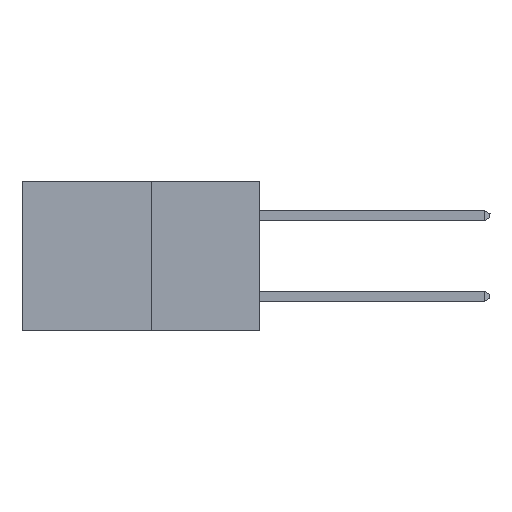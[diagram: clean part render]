
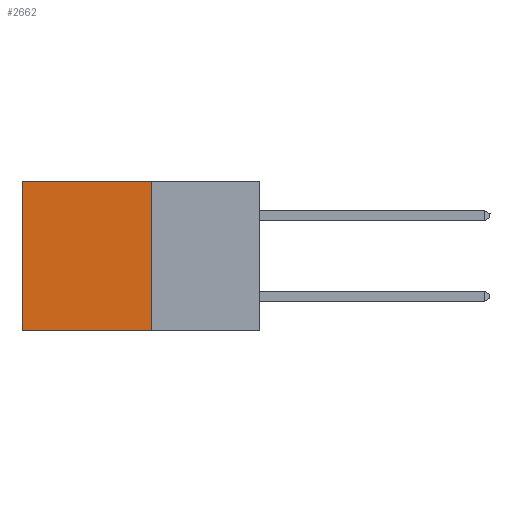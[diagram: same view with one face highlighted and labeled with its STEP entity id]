
A CAD part, left-side view. The second image highlights one B-rep face of the part: STEP entity #2662.
In plain terms, the highlighted planar face has unit normal (-1, 0, 0).
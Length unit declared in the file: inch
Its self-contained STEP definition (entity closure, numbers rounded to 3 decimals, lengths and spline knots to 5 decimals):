
#34 = EDGE_CURVE ( 'NONE', #8551, #8458, #6924, .T. ) ;
#679 = DIRECTION ( 'NONE',  ( 0., 1., 0. ) ) ;
#1258 = CARTESIAN_POINT ( 'NONE',  ( 0.277, 0.27, -0.37 ) ) ;
#1475 = CARTESIAN_POINT ( 'NONE',  ( 0.277, 0.27, -0.37 ) ) ;
#1746 = EDGE_CURVE ( 'NONE', #8458, #3510, #6960, .T. ) ;
#2033 = CARTESIAN_POINT ( 'NONE',  ( 0.277, 0.27, 0. ) ) ;
#2217 = CARTESIAN_POINT ( 'NONE',  ( 0.277, 0.27, 0. ) ) ;
#2527 = VECTOR ( 'NONE', #5735, 39.37008 ) ;
#2662 = ADVANCED_FACE ( 'NONE', ( #6416 ), #9100, .F. ) ;
#3169 = CARTESIAN_POINT ( 'NONE',  ( 0.277, 0.59, -0.37 ) ) ;
#3482 = AXIS2_PLACEMENT_3D ( 'NONE', #1258, #4372, #9853 ) ;
#3510 = VERTEX_POINT ( 'NONE', #3169 ) ;
#3789 = CARTESIAN_POINT ( 'NONE',  ( 0.277, 0.27, -0.37 ) ) ;
#4079 = EDGE_CURVE ( 'NONE', #4825, #3510, #6395, .T. ) ;
#4168 = EDGE_LOOP ( 'NONE', ( #6909, #8993, #7153, #9236 ) ) ;
#4241 = CARTESIAN_POINT ( 'NONE',  ( 0.277, 0.59, 0. ) ) ;
#4372 = DIRECTION ( 'NONE',  ( 1., 0., 0. ) ) ;
#4825 = VERTEX_POINT ( 'NONE', #9370 ) ;
#5362 = DIRECTION ( 'NONE',  ( 0., 0., -1. ) ) ;
#5722 = CARTESIAN_POINT ( 'NONE',  ( 0.277, 0.59, -0.37 ) ) ;
#5735 = DIRECTION ( 'NONE',  ( 0., 1., 0. ) ) ;
#6162 = DIRECTION ( 'NONE',  ( 0., 0., -1. ) ) ;
#6178 = EDGE_CURVE ( 'NONE', #8551, #4825, #7381, .T. ) ;
#6395 = LINE ( 'NONE', #1475, #8261 ) ;
#6416 = FACE_OUTER_BOUND ( 'NONE', #4168, .T. ) ;
#6909 = ORIENTED_EDGE ( 'NONE', *, *, #1746, .T. ) ;
#6924 = LINE ( 'NONE', #2217, #2527 ) ;
#6960 = LINE ( 'NONE', #5722, #9047 ) ;
#7135 = VECTOR ( 'NONE', #6162, 39.37008 ) ;
#7153 = ORIENTED_EDGE ( 'NONE', *, *, #6178, .F. ) ;
#7381 = LINE ( 'NONE', #3789, #7135 ) ;
#8261 = VECTOR ( 'NONE', #679, 39.37008 ) ;
#8458 = VERTEX_POINT ( 'NONE', #4241 ) ;
#8551 = VERTEX_POINT ( 'NONE', #2033 ) ;
#8993 = ORIENTED_EDGE ( 'NONE', *, *, #4079, .F. ) ;
#9047 = VECTOR ( 'NONE', #5362, 39.37008 ) ;
#9100 = PLANE ( 'NONE',  #3482 ) ;
#9236 = ORIENTED_EDGE ( 'NONE', *, *, #34, .T. ) ;
#9370 = CARTESIAN_POINT ( 'NONE',  ( 0.277, 0.27, -0.37 ) ) ;
#9853 = DIRECTION ( 'NONE',  ( 0., 0., -1. ) ) ;
